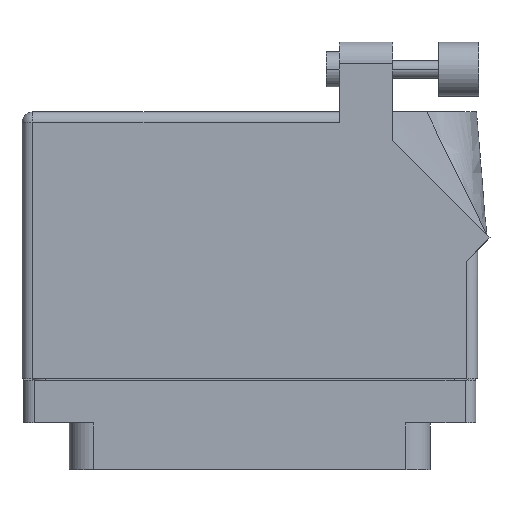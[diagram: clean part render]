
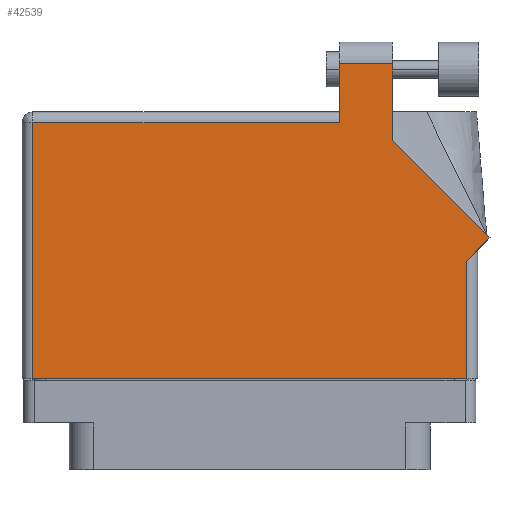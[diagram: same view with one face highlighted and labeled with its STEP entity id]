
A CAD part, front view. The second image highlights one B-rep face of the part: STEP entity #42539.
In plain terms, the highlighted face is planar.
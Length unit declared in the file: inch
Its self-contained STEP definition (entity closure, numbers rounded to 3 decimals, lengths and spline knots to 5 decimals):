
#113 = CARTESIAN_POINT ( 'NONE',  ( 0.82, 1.26442, 0.455 ) ) ;
#375 = CARTESIAN_POINT ( 'NONE',  ( 0.513, 1.705, 0.455 ) ) ;
#819 = CARTESIAN_POINT ( 'NONE',  ( -1.306, 1.368, 0.455 ) ) ;
#960 = ORIENTED_EDGE ( 'NONE', *, *, #18870, .T. ) ;
#2853 = VECTOR ( 'NONE', #9812, 39.37008 ) ;
#3532 = VERTEX_POINT ( 'NONE', #22781 ) ;
#4110 = CARTESIAN_POINT ( 'NONE',  ( 0.82, 1.26442, 0.455 ) ) ;
#4277 = DIRECTION ( 'NONE',  ( -1., 0., 0. ) ) ;
#4462 = DIRECTION ( 'NONE',  ( -0.707, 0.707, 0. ) ) ;
#4941 = CARTESIAN_POINT ( 'NONE',  ( 1.244, 0.637, 0.455 ) ) ;
#5204 = LINE ( 'NONE', #5663, #34632 ) ;
#5441 = DIRECTION ( 'NONE',  ( 0., -1., 0. ) ) ;
#5663 = CARTESIAN_POINT ( 'NONE',  ( -1.244, -0.1, 0.455 ) ) ;
#6570 = VERTEX_POINT ( 'NONE', #39640 ) ;
#7384 = EDGE_CURVE ( 'NONE', #37992, #3532, #17141, .T. ) ;
#8230 = VECTOR ( 'NONE', #4277, 39.37008 ) ;
#9519 = LINE ( 'NONE', #22845, #21101 ) ;
#9574 = DIRECTION ( 'NONE',  ( 0., 0., -1. ) ) ;
#9812 = DIRECTION ( 'NONE',  ( 0.707, 0.707, 0. ) ) ;
#9832 = VECTOR ( 'NONE', #47761, 39.37008 ) ;
#9930 = VERTEX_POINT ( 'NONE', #4110 ) ;
#11212 = EDGE_CURVE ( 'NONE', #47634, #6570, #41407, .T. ) ;
#11371 = VECTOR ( 'NONE', #12300, 39.37008 ) ;
#12300 = DIRECTION ( 'NONE',  ( 1., 0., 0. ) ) ;
#12318 = VERTEX_POINT ( 'NONE', #42091 ) ;
#13344 = EDGE_LOOP ( 'NONE', ( #42113, #17263, #33855, #29298, #24041, #16765, #18628, #36325, #960 ) ) ;
#13912 = EDGE_CURVE ( 'NONE', #6570, #29588, #19827, .T. ) ;
#14399 = FACE_OUTER_BOUND ( 'NONE', #13344, .T. ) ;
#14457 = CARTESIAN_POINT ( 'NONE',  ( 1.37671, 0.70771, 0.455 ) ) ;
#16091 = CARTESIAN_POINT ( 'NONE',  ( 0.513, 1.368, 0.455 ) ) ;
#16765 = ORIENTED_EDGE ( 'NONE', *, *, #11212, .T. ) ;
#17141 = LINE ( 'NONE', #819, #20024 ) ;
#17263 = ORIENTED_EDGE ( 'NONE', *, *, #28325, .T. ) ;
#18342 = VERTEX_POINT ( 'NONE', #14457 ) ;
#18628 = ORIENTED_EDGE ( 'NONE', *, *, #13912, .T. ) ;
#18870 = EDGE_CURVE ( 'NONE', #18342, #9930, #9519, .T. ) ;
#19219 = AXIS2_PLACEMENT_3D ( 'NONE', #28284, #9574, #46402 ) ;
#19827 = LINE ( 'NONE', #4941, #36547 ) ;
#20024 = VECTOR ( 'NONE', #45674, 39.37008 ) ;
#20723 = DIRECTION ( 'NONE',  ( 0., 1., 0. ) ) ;
#21101 = VECTOR ( 'NONE', #4462, 39.37008 ) ;
#22079 = LINE ( 'NONE', #375, #8230 ) ;
#22477 = LINE ( 'NONE', #35492, #2853 ) ;
#22781 = CARTESIAN_POINT ( 'NONE',  ( -1.244, 1.368, 0.455 ) ) ;
#22845 = CARTESIAN_POINT ( 'NONE',  ( 1.37671, 0.70771, 0.455 ) ) ;
#22859 = VECTOR ( 'NONE', #5441, 39.37008 ) ;
#24041 = ORIENTED_EDGE ( 'NONE', *, *, #37515, .T. ) ;
#24096 = CARTESIAN_POINT ( 'NONE',  ( 1.244, 0.575, 0.455 ) ) ;
#27900 = DIRECTION ( 'NONE',  ( 0., -1., 0. ) ) ;
#28284 = CARTESIAN_POINT ( 'NONE',  ( -1.306, 1.43, 0.455 ) ) ;
#28325 = EDGE_CURVE ( 'NONE', #47309, #12318, #22079, .T. ) ;
#28927 = CARTESIAN_POINT ( 'NONE',  ( 0.82, 1.705, 0.455 ) ) ;
#29298 = ORIENTED_EDGE ( 'NONE', *, *, #7384, .T. ) ;
#29588 = VERTEX_POINT ( 'NONE', #24096 ) ;
#33855 = ORIENTED_EDGE ( 'NONE', *, *, #45294, .T. ) ;
#34235 = CARTESIAN_POINT ( 'NONE',  ( -1.306, -0.1, 0.455 ) ) ;
#34241 = CARTESIAN_POINT ( 'NONE',  ( -1.244, -0.1, 0.455 ) ) ;
#34632 = VECTOR ( 'NONE', #27900, 39.37008 ) ;
#35492 = CARTESIAN_POINT ( 'NONE',  ( 1.306, 0.637, 0.455 ) ) ;
#36325 = ORIENTED_EDGE ( 'NONE', *, *, #41703, .T. ) ;
#36547 = VECTOR ( 'NONE', #20723, 39.37008 ) ;
#37006 = LINE ( 'NONE', #113, #9832 ) ;
#37515 = EDGE_CURVE ( 'NONE', #3532, #47634, #5204, .T. ) ;
#37992 = VERTEX_POINT ( 'NONE', #16091 ) ;
#39297 = PLANE ( 'NONE',  #19219 ) ;
#39640 = CARTESIAN_POINT ( 'NONE',  ( 1.244, -0.1, 0.455 ) ) ;
#40767 = LINE ( 'NONE', #42684, #22859 ) ;
#40994 = EDGE_CURVE ( 'NONE', #9930, #47309, #37006, .T. ) ;
#41407 = LINE ( 'NONE', #34235, #11371 ) ;
#41703 = EDGE_CURVE ( 'NONE', #29588, #18342, #22477, .T. ) ;
#42091 = CARTESIAN_POINT ( 'NONE',  ( 0.513, 1.705, 0.455 ) ) ;
#42113 = ORIENTED_EDGE ( 'NONE', *, *, #40994, .T. ) ;
#42539 = ADVANCED_FACE ( 'NONE', ( #14399 ), #39297, .F. ) ;
#42684 = CARTESIAN_POINT ( 'NONE',  ( 0.513, 1.43, 0.455 ) ) ;
#45294 = EDGE_CURVE ( 'NONE', #12318, #37992, #40767, .T. ) ;
#45674 = DIRECTION ( 'NONE',  ( -1., 0., 0. ) ) ;
#46402 = DIRECTION ( 'NONE',  ( -1., 0., 0. ) ) ;
#47309 = VERTEX_POINT ( 'NONE', #28927 ) ;
#47634 = VERTEX_POINT ( 'NONE', #34241 ) ;
#47761 = DIRECTION ( 'NONE',  ( 0., 1., 0. ) ) ;
